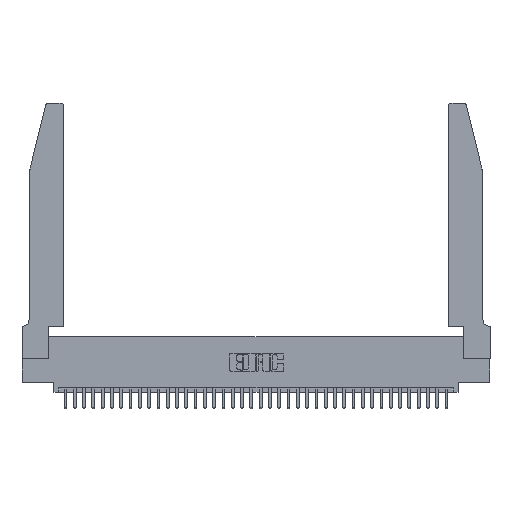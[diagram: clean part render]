
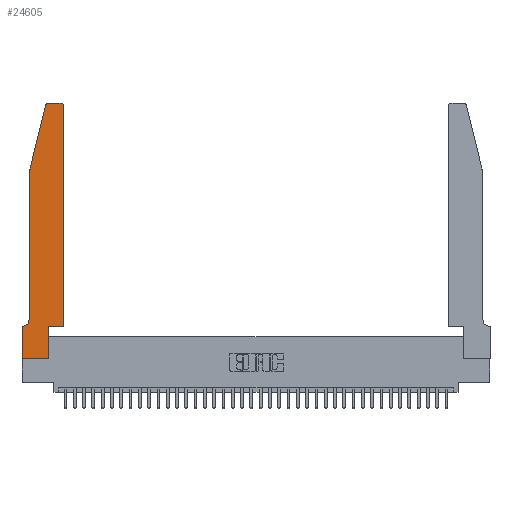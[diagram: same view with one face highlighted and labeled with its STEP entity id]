
A CAD part, top view. The second image highlights one B-rep face of the part: STEP entity #24605.
In plain terms, the highlighted planar face has unit normal (0, 0, 1).
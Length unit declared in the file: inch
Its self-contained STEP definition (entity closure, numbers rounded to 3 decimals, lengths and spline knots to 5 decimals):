
#202 = CARTESIAN_POINT ( 'NONE',  ( 0.0755, 2., 0.37 ) ) ;
#536 = LINE ( 'NONE', #7035, #3326 ) ;
#619 = VECTOR ( 'NONE', #35001, 39.37008 ) ;
#642 = EDGE_CURVE ( 'NONE', #9588, #11507, #536, .T. ) ;
#2373 = ORIENTED_EDGE ( 'NONE', *, *, #642, .T. ) ;
#2527 = DIRECTION ( 'NONE',  ( 0., 0., 1. ) ) ;
#3272 = CIRCLE ( 'NONE', #23308, 0.03 ) ;
#3326 = VECTOR ( 'NONE', #11004, 39.37008 ) ;
#4176 = ORIENTED_EDGE ( 'NONE', *, *, #7325, .T. ) ;
#4884 = VERTEX_POINT ( 'NONE', #35647 ) ;
#5253 = CARTESIAN_POINT ( 'NONE',  ( 0.2865, 0.35, 0.37 ) ) ;
#5567 = DIRECTION ( 'NONE',  ( 1., 0., 0. ) ) ;
#5729 = CARTESIAN_POINT ( 'NONE',  ( 0.0755, 0.35, 0.37 ) ) ;
#5949 = VECTOR ( 'NONE', #36157, 39.37008 ) ;
#6842 = FACE_OUTER_BOUND ( 'NONE', #24617, .T. ) ;
#6855 = EDGE_CURVE ( 'NONE', #8027, #4884, #20867, .T. ) ;
#7035 = CARTESIAN_POINT ( 'NONE',  ( 0.2605, 2.75, 0.37 ) ) ;
#7280 = VERTEX_POINT ( 'NONE', #23808 ) ;
#7311 = CARTESIAN_POINT ( 'NONE',  ( 0.2865, 0.35, 0.37 ) ) ;
#7325 = EDGE_CURVE ( 'NONE', #7485, #9588, #15727, .T. ) ;
#7485 = VERTEX_POINT ( 'NONE', #9270 ) ;
#7504 = DIRECTION ( 'NONE',  ( 0., -1., 0. ) ) ;
#7818 = PLANE ( 'NONE',  #11882 ) ;
#8027 = VERTEX_POINT ( 'NONE', #11078 ) ;
#8588 = CARTESIAN_POINT ( 'NONE',  ( 0.4505, 0.35, 0.37 ) ) ;
#8675 = DIRECTION ( 'NONE',  ( -1., 0., 0. ) ) ;
#8836 = DIRECTION ( 'NONE',  ( 1., 0., 0. ) ) ;
#9270 = CARTESIAN_POINT ( 'NONE',  ( 0.4505, 2.72, 0.37 ) ) ;
#9550 = DIRECTION ( 'NONE',  ( 1., 0., 0. ) ) ;
#9588 = VERTEX_POINT ( 'NONE', #18737 ) ;
#9881 = VERTEX_POINT ( 'NONE', #5253 ) ;
#10951 = ORIENTED_EDGE ( 'NONE', *, *, #6855, .T. ) ;
#11004 = DIRECTION ( 'NONE',  ( -1., 0., 0. ) ) ;
#11078 = CARTESIAN_POINT ( 'NONE',  ( 0.0755, 2., 0.37 ) ) ;
#11507 = VERTEX_POINT ( 'NONE', #30933 ) ;
#11882 = AXIS2_PLACEMENT_3D ( 'NONE', #25849, #2527, #37114 ) ;
#12088 = CARTESIAN_POINT ( 'NONE',  ( 0.25487, 2.72718, 0.37 ) ) ;
#12330 = CARTESIAN_POINT ( 'NONE',  ( 0.2865, 0., 0.37 ) ) ;
#12404 = LINE ( 'NONE', #37385, #25702 ) ;
#12501 = ORIENTED_EDGE ( 'NONE', *, *, #16120, .T. ) ;
#12924 = VECTOR ( 'NONE', #8836, 39.37008 ) ;
#14595 = DIRECTION ( 'NONE',  ( -1., 0., 0. ) ) ;
#14638 = EDGE_CURVE ( 'NONE', #34338, #8027, #12404, .T. ) ;
#14666 = CARTESIAN_POINT ( 'NONE',  ( 0.0055, 0.35, 0.37 ) ) ;
#14818 = VECTOR ( 'NONE', #22985, 39.37008 ) ;
#15012 = CARTESIAN_POINT ( 'NONE',  ( 0., 0.35, 0.37 ) ) ;
#15727 = CIRCLE ( 'NONE', #34187, 0.03 ) ;
#15958 = EDGE_CURVE ( 'NONE', #25468, #7280, #20793, .T. ) ;
#16113 = LINE ( 'NONE', #8588, #12924 ) ;
#16120 = EDGE_CURVE ( 'NONE', #37776, #7485, #24892, .T. ) ;
#18132 = CARTESIAN_POINT ( 'NONE',  ( 0.284, 2.72, 0.37 ) ) ;
#18380 = CARTESIAN_POINT ( 'NONE',  ( 0., 0., 0.37 ) ) ;
#18737 = CARTESIAN_POINT ( 'NONE',  ( 0.4205, 2.75, 0.37 ) ) ;
#18889 = VERTEX_POINT ( 'NONE', #14666 ) ;
#19192 = EDGE_CURVE ( 'NONE', #7280, #30191, #19234, .T. ) ;
#19234 = LINE ( 'NONE', #18380, #5949 ) ;
#20793 = LINE ( 'NONE', #25054, #34991 ) ;
#20867 = LINE ( 'NONE', #202, #619 ) ;
#22983 = CIRCLE ( 'NONE', #24541, 0.07 ) ;
#22985 = DIRECTION ( 'NONE',  ( 0., 1., 0. ) ) ;
#23192 = DIRECTION ( 'NONE',  ( 0., 1., 0. ) ) ;
#23308 = AXIS2_PLACEMENT_3D ( 'NONE', #18132, #32961, #9550 ) ;
#23677 = DIRECTION ( 'NONE',  ( 0., 0., -1. ) ) ;
#23808 = CARTESIAN_POINT ( 'NONE',  ( 0., 0., 0.37 ) ) ;
#24028 = EDGE_CURVE ( 'NONE', #30191, #9881, #32079, .T. ) ;
#24541 = AXIS2_PLACEMENT_3D ( 'NONE', #32140, #23677, #14595 ) ;
#24605 = ADVANCED_FACE ( 'NONE', ( #6842 ), #7818, .T. ) ;
#24617 = EDGE_LOOP ( 'NONE', ( #2373, #32761, #31754, #10951, #26477, #36924, #29002, #28898, #31314, #29987, #12501, #4176 ) ) ;
#24766 = VECTOR ( 'NONE', #23192, 39.37008 ) ;
#24892 = LINE ( 'NONE', #34500, #14818 ) ;
#25054 = CARTESIAN_POINT ( 'NONE',  ( 0., 0., 0.37 ) ) ;
#25468 = VERTEX_POINT ( 'NONE', #15012 ) ;
#25702 = VECTOR ( 'NONE', #34697, 39.37008 ) ;
#25849 = CARTESIAN_POINT ( 'NONE',  ( 0., 0.35, 0.37 ) ) ;
#26477 = ORIENTED_EDGE ( 'NONE', *, *, #30735, .T. ) ;
#27107 = VECTOR ( 'NONE', #8675, 39.37008 ) ;
#28649 = DIRECTION ( 'NONE',  ( 0., 0., 1. ) ) ;
#28898 = ORIENTED_EDGE ( 'NONE', *, *, #19192, .T. ) ;
#28959 = LINE ( 'NONE', #5729, #27107 ) ;
#29000 = CARTESIAN_POINT ( 'NONE',  ( 0.4505, 0.35, 0.37 ) ) ;
#29002 = ORIENTED_EDGE ( 'NONE', *, *, #15958, .T. ) ;
#29987 = ORIENTED_EDGE ( 'NONE', *, *, #30604, .T. ) ;
#30191 = VERTEX_POINT ( 'NONE', #12330 ) ;
#30604 = EDGE_CURVE ( 'NONE', #9881, #37776, #16113, .T. ) ;
#30735 = EDGE_CURVE ( 'NONE', #4884, #18889, #22983, .T. ) ;
#30933 = CARTESIAN_POINT ( 'NONE',  ( 0.284, 2.75, 0.37 ) ) ;
#31314 = ORIENTED_EDGE ( 'NONE', *, *, #24028, .T. ) ;
#31574 = EDGE_CURVE ( 'NONE', #11507, #34338, #3272, .T. ) ;
#31754 = ORIENTED_EDGE ( 'NONE', *, *, #14638, .T. ) ;
#32079 = LINE ( 'NONE', #7311, #24766 ) ;
#32140 = CARTESIAN_POINT ( 'NONE',  ( 0.0055, 0.42, 0.37 ) ) ;
#32761 = ORIENTED_EDGE ( 'NONE', *, *, #31574, .T. ) ;
#32961 = DIRECTION ( 'NONE',  ( 0., 0., 1. ) ) ;
#34187 = AXIS2_PLACEMENT_3D ( 'NONE', #35011, #28649, #5567 ) ;
#34338 = VERTEX_POINT ( 'NONE', #12088 ) ;
#34500 = CARTESIAN_POINT ( 'NONE',  ( 0.4505, 0.35, 0.37 ) ) ;
#34697 = DIRECTION ( 'NONE',  ( -0.239, -0.971, 0. ) ) ;
#34991 = VECTOR ( 'NONE', #7504, 39.37008 ) ;
#35001 = DIRECTION ( 'NONE',  ( 0., -1., 0. ) ) ;
#35011 = CARTESIAN_POINT ( 'NONE',  ( 0.4205, 2.72, 0.37 ) ) ;
#35647 = CARTESIAN_POINT ( 'NONE',  ( 0.0755, 0.42, 0.37 ) ) ;
#36157 = DIRECTION ( 'NONE',  ( 1., 0., 0. ) ) ;
#36924 = ORIENTED_EDGE ( 'NONE', *, *, #37083, .T. ) ;
#37083 = EDGE_CURVE ( 'NONE', #18889, #25468, #28959, .T. ) ;
#37114 = DIRECTION ( 'NONE',  ( 1., 0., 0. ) ) ;
#37385 = CARTESIAN_POINT ( 'NONE',  ( 0.0755, 2., 0.37 ) ) ;
#37776 = VERTEX_POINT ( 'NONE', #29000 ) ;
